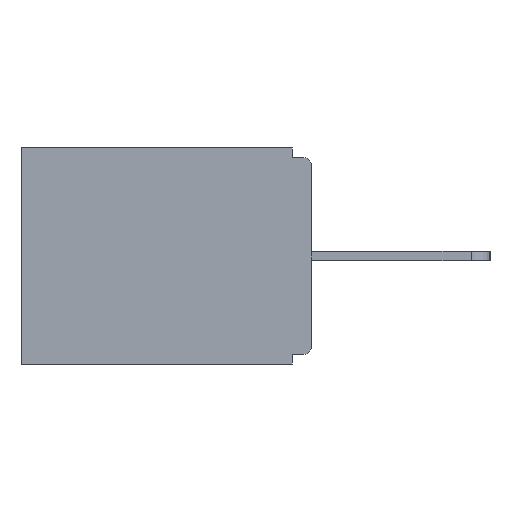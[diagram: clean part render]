
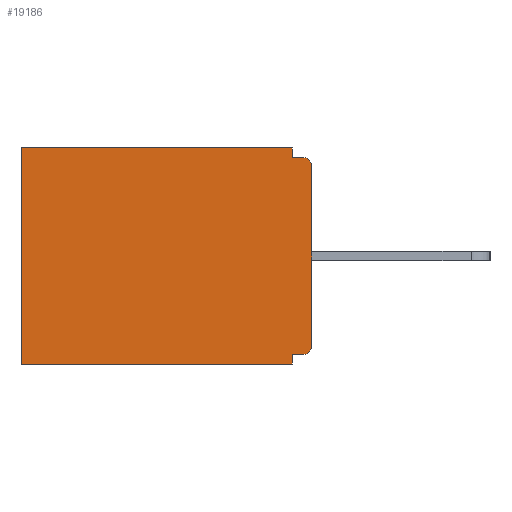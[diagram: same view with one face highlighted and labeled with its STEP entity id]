
A CAD part, left-side view. The second image highlights one B-rep face of the part: STEP entity #19186.
In plain terms, the highlighted planar face has unit normal (-1, 0, 0).
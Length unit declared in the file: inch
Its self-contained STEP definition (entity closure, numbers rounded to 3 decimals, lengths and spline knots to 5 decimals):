
#88 = EDGE_CURVE ( 'NONE', #13295, #20840, #12688, .T. ) ;
#630 = EDGE_LOOP ( 'NONE', ( #793, #8154, #1428, #21425, #16365, #19976, #15836, #8614, #13181, #10468 ) ) ;
#644 = AXIS2_PLACEMENT_3D ( 'NONE', #8413, #1914, #17170 ) ;
#793 = ORIENTED_EDGE ( 'NONE', *, *, #3415, .T. ) ;
#848 = CARTESIAN_POINT ( 'NONE',  ( 0.298, 0.46, 0. ) ) ;
#1153 = CARTESIAN_POINT ( 'NONE',  ( 0.298, 0., -0.328 ) ) ;
#1206 = VERTEX_POINT ( 'NONE', #21256 ) ;
#1279 = VERTEX_POINT ( 'NONE', #17551 ) ;
#1428 = ORIENTED_EDGE ( 'NONE', *, *, #13784, .F. ) ;
#1914 = DIRECTION ( 'NONE',  ( -1., 0., 0. ) ) ;
#2203 = CARTESIAN_POINT ( 'NONE',  ( 0.298, 0., 0. ) ) ;
#2620 = CARTESIAN_POINT ( 'NONE',  ( 0.298, 0.031, -0.015 ) ) ;
#3223 = LINE ( 'NONE', #21836, #6208 ) ;
#3415 = EDGE_CURVE ( 'NONE', #1279, #1206, #10343, .T. ) ;
#3778 = DIRECTION ( 'NONE',  ( 0., 0., -1. ) ) ;
#4209 = LINE ( 'NONE', #19321, #9084 ) ;
#4505 = VECTOR ( 'NONE', #5951, 39.37008 ) ;
#4639 = CARTESIAN_POINT ( 'NONE',  ( 0.298, 0., -0.313 ) ) ;
#5283 = EDGE_CURVE ( 'NONE', #12327, #13295, #12519, .T. ) ;
#5449 = EDGE_CURVE ( 'NONE', #13050, #18914, #19342, .T. ) ;
#5643 = DIRECTION ( 'NONE',  ( 0., 0., -1. ) ) ;
#5936 = DIRECTION ( 'NONE',  ( 1., 0., 0. ) ) ;
#5951 = DIRECTION ( 'NONE',  ( 0., 0., -1. ) ) ;
#6084 = CARTESIAN_POINT ( 'NONE',  ( 0.298, 0.031, -0.343 ) ) ;
#6208 = VECTOR ( 'NONE', #14628, 39.37008 ) ;
#7396 = CARTESIAN_POINT ( 'NONE',  ( 0.298, 0.031, -0.328 ) ) ;
#7402 = CARTESIAN_POINT ( 'NONE',  ( 0.298, 0., 0. ) ) ;
#8154 = ORIENTED_EDGE ( 'NONE', *, *, #13449, .F. ) ;
#8413 = CARTESIAN_POINT ( 'NONE',  ( 0.298, 0.015, -0.03 ) ) ;
#8614 = ORIENTED_EDGE ( 'NONE', *, *, #18876, .F. ) ;
#9084 = VECTOR ( 'NONE', #9243, 39.37008 ) ;
#9243 = DIRECTION ( 'NONE',  ( 0., 0., -1. ) ) ;
#9382 = LINE ( 'NONE', #6084, #11657 ) ;
#10277 = CARTESIAN_POINT ( 'NONE',  ( 0.298, 0.031, 0. ) ) ;
#10343 = CIRCLE ( 'NONE', #644, 0.015 ) ;
#10468 = ORIENTED_EDGE ( 'NONE', *, *, #21814, .F. ) ;
#11017 = VECTOR ( 'NONE', #3778, 39.37008 ) ;
#11219 = PLANE ( 'NONE',  #12064 ) ;
#11657 = VECTOR ( 'NONE', #5643, 39.37008 ) ;
#11810 = LINE ( 'NONE', #1153, #20993 ) ;
#11916 = DIRECTION ( 'NONE',  ( 0., 1., 0. ) ) ;
#12064 = AXIS2_PLACEMENT_3D ( 'NONE', #7402, #5936, #12793 ) ;
#12327 = VERTEX_POINT ( 'NONE', #10277 ) ;
#12519 = LINE ( 'NONE', #2203, #17752 ) ;
#12621 = LINE ( 'NONE', #17890, #11017 ) ;
#12688 = LINE ( 'NONE', #19876, #4505 ) ;
#12793 = DIRECTION ( 'NONE',  ( 0., 0., -1. ) ) ;
#13050 = VERTEX_POINT ( 'NONE', #18151 ) ;
#13181 = ORIENTED_EDGE ( 'NONE', *, *, #5449, .T. ) ;
#13281 = AXIS2_PLACEMENT_3D ( 'NONE', #14973, #18684, #20275 ) ;
#13295 = VERTEX_POINT ( 'NONE', #848 ) ;
#13449 = EDGE_CURVE ( 'NONE', #20060, #1206, #3223, .T. ) ;
#13784 = EDGE_CURVE ( 'NONE', #12327, #20060, #4209, .T. ) ;
#14494 = CARTESIAN_POINT ( 'NONE',  ( 0.298, 0., -0.343 ) ) ;
#14628 = DIRECTION ( 'NONE',  ( 0., -1., 0. ) ) ;
#14671 = FACE_OUTER_BOUND ( 'NONE', #630, .T. ) ;
#14973 = CARTESIAN_POINT ( 'NONE',  ( 0.298, 0.015, -0.313 ) ) ;
#15244 = VERTEX_POINT ( 'NONE', #21783 ) ;
#15374 = CARTESIAN_POINT ( 'NONE',  ( 0.298, 0.46, -0.343 ) ) ;
#15836 = ORIENTED_EDGE ( 'NONE', *, *, #16250, .F. ) ;
#15848 = EDGE_CURVE ( 'NONE', #15244, #20840, #17547, .T. ) ;
#16250 = EDGE_CURVE ( 'NONE', #20984, #15244, #9382, .T. ) ;
#16365 = ORIENTED_EDGE ( 'NONE', *, *, #88, .T. ) ;
#17170 = DIRECTION ( 'NONE',  ( 0., 0., -1. ) ) ;
#17547 = LINE ( 'NONE', #14494, #22037 ) ;
#17551 = CARTESIAN_POINT ( 'NONE',  ( 0.298, 0., -0.03 ) ) ;
#17752 = VECTOR ( 'NONE', #19348, 39.37008 ) ;
#17890 = CARTESIAN_POINT ( 'NONE',  ( 0.298, 0., 0. ) ) ;
#18151 = CARTESIAN_POINT ( 'NONE',  ( 0.298, 0.015, -0.328 ) ) ;
#18684 = DIRECTION ( 'NONE',  ( -1., 0., 0. ) ) ;
#18876 = EDGE_CURVE ( 'NONE', #13050, #20984, #11810, .T. ) ;
#18914 = VERTEX_POINT ( 'NONE', #4639 ) ;
#19186 = ADVANCED_FACE ( 'NONE', ( #14671 ), #11219, .F. ) ;
#19321 = CARTESIAN_POINT ( 'NONE',  ( 0.298, 0.031, -0.343 ) ) ;
#19342 = CIRCLE ( 'NONE', #13281, 0.015 ) ;
#19348 = DIRECTION ( 'NONE',  ( 0., 1., 0. ) ) ;
#19876 = CARTESIAN_POINT ( 'NONE',  ( 0.298, 0.46, 0. ) ) ;
#19976 = ORIENTED_EDGE ( 'NONE', *, *, #15848, .F. ) ;
#20060 = VERTEX_POINT ( 'NONE', #2620 ) ;
#20275 = DIRECTION ( 'NONE',  ( 0., 0., -1. ) ) ;
#20840 = VERTEX_POINT ( 'NONE', #15374 ) ;
#20984 = VERTEX_POINT ( 'NONE', #7396 ) ;
#20993 = VECTOR ( 'NONE', #11916, 39.37008 ) ;
#21252 = DIRECTION ( 'NONE',  ( 0., 1., 0. ) ) ;
#21256 = CARTESIAN_POINT ( 'NONE',  ( 0.298, 0.015, -0.015 ) ) ;
#21425 = ORIENTED_EDGE ( 'NONE', *, *, #5283, .T. ) ;
#21783 = CARTESIAN_POINT ( 'NONE',  ( 0.298, 0.031, -0.343 ) ) ;
#21814 = EDGE_CURVE ( 'NONE', #1279, #18914, #12621, .T. ) ;
#21836 = CARTESIAN_POINT ( 'NONE',  ( 0.298, 0., -0.015 ) ) ;
#22037 = VECTOR ( 'NONE', #21252, 39.37008 ) ;
